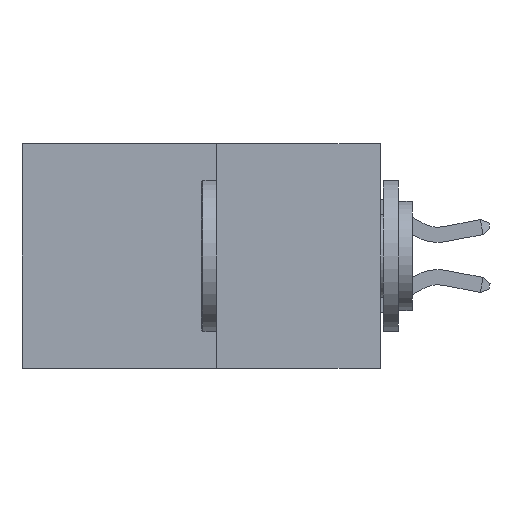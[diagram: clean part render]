
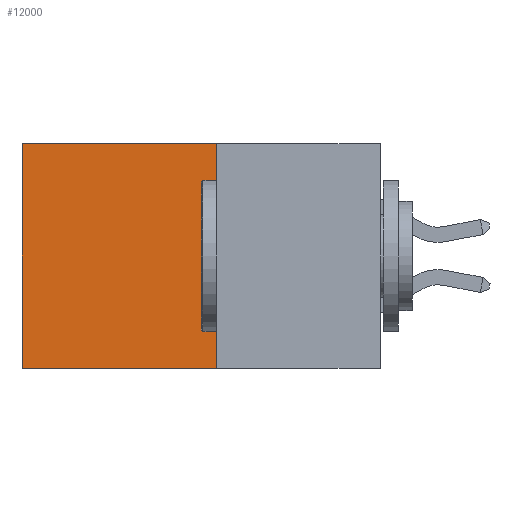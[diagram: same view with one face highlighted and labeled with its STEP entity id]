
A CAD part, left-side view. The second image highlights one B-rep face of the part: STEP entity #12000.
In plain terms, the highlighted planar face has unit normal (-1, 0, 0).
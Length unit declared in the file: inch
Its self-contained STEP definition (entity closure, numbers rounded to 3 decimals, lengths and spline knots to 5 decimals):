
#30 = DIRECTION ( 'NONE',  ( 0., 1., 0. ) ) ;
#337 = DIRECTION ( 'NONE',  ( 0., 0., -1. ) ) ;
#463 = CARTESIAN_POINT ( 'NONE',  ( 0.277, 0.27, -0.37 ) ) ;
#992 = ORIENTED_EDGE ( 'NONE', *, *, #8099, .F. ) ;
#1629 = CARTESIAN_POINT ( 'NONE',  ( 0.277, 0.27, -0.37 ) ) ;
#2011 = ORIENTED_EDGE ( 'NONE', *, *, #10516, .F. ) ;
#2211 = CARTESIAN_POINT ( 'NONE',  ( 0.277, 0.27, -0.37 ) ) ;
#2426 = VECTOR ( 'NONE', #15027, 39.37008 ) ;
#3187 = LINE ( 'NONE', #13655, #9332 ) ;
#3693 = DIRECTION ( 'NONE',  ( 0., 1., 0. ) ) ;
#3701 = CARTESIAN_POINT ( 'NONE',  ( 0.277, 0.27, 0. ) ) ;
#3771 = ORIENTED_EDGE ( 'NONE', *, *, #15926, .T. ) ;
#3835 = VERTEX_POINT ( 'NONE', #3701 ) ;
#3878 = VECTOR ( 'NONE', #337, 39.37008 ) ;
#4014 = CARTESIAN_POINT ( 'NONE',  ( 0.277, 0.59, -0.37 ) ) ;
#4279 = LINE ( 'NONE', #463, #3878 ) ;
#5734 = LINE ( 'NONE', #4014, #2426 ) ;
#6384 = VERTEX_POINT ( 'NONE', #13329 ) ;
#6623 = DIRECTION ( 'NONE',  ( 0., 0., -1. ) ) ;
#6778 = CARTESIAN_POINT ( 'NONE',  ( 0.277, 0.59, 0. ) ) ;
#7333 = EDGE_LOOP ( 'NONE', ( #3771, #2011, #992, #8398 ) ) ;
#8099 = EDGE_CURVE ( 'NONE', #3835, #13109, #4279, .T. ) ;
#8398 = ORIENTED_EDGE ( 'NONE', *, *, #15266, .T. ) ;
#9332 = VECTOR ( 'NONE', #30, 39.37008 ) ;
#9575 = VECTOR ( 'NONE', #3693, 39.37008 ) ;
#10516 = EDGE_CURVE ( 'NONE', #13109, #6384, #3187, .T. ) ;
#12000 = ADVANCED_FACE ( 'NONE', ( #13498 ), #12754, .F. ) ;
#12754 = PLANE ( 'NONE',  #14222 ) ;
#13109 = VERTEX_POINT ( 'NONE', #2211 ) ;
#13329 = CARTESIAN_POINT ( 'NONE',  ( 0.277, 0.59, -0.37 ) ) ;
#13498 = FACE_OUTER_BOUND ( 'NONE', #7333, .T. ) ;
#13619 = VERTEX_POINT ( 'NONE', #6778 ) ;
#13655 = CARTESIAN_POINT ( 'NONE',  ( 0.277, 0.27, -0.37 ) ) ;
#13989 = DIRECTION ( 'NONE',  ( 1., 0., 0. ) ) ;
#14222 = AXIS2_PLACEMENT_3D ( 'NONE', #1629, #13989, #6623 ) ;
#14667 = CARTESIAN_POINT ( 'NONE',  ( 0.277, 0.27, 0. ) ) ;
#15027 = DIRECTION ( 'NONE',  ( 0., 0., -1. ) ) ;
#15266 = EDGE_CURVE ( 'NONE', #3835, #13619, #15661, .T. ) ;
#15661 = LINE ( 'NONE', #14667, #9575 ) ;
#15926 = EDGE_CURVE ( 'NONE', #13619, #6384, #5734, .T. ) ;
